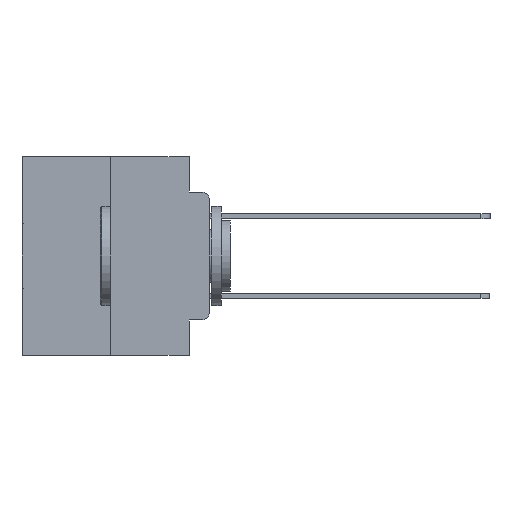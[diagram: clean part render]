
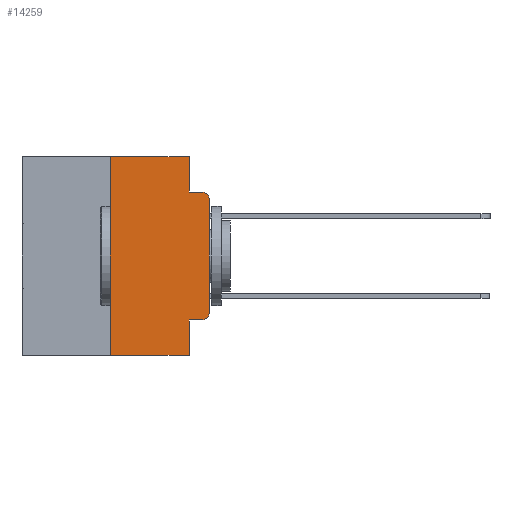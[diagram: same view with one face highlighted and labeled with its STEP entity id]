
A CAD part, left-side view. The second image highlights one B-rep face of the part: STEP entity #14259.
In plain terms, the highlighted planar face has unit normal (-1, 0, 0).
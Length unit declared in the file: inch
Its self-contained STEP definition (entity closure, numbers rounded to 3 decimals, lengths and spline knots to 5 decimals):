
#190 = LINE ( 'NONE', #10588, #1697 ) ;
#685 = CARTESIAN_POINT ( 'NONE',  ( 0., 0.051, -0.0885 ) ) ;
#853 = VERTEX_POINT ( 'NONE', #22486 ) ;
#1015 = EDGE_CURVE ( 'NONE', #21438, #19655, #23210, .T. ) ;
#1168 = VERTEX_POINT ( 'NONE', #1882 ) ;
#1697 = VECTOR ( 'NONE', #24722, 39.37008 ) ;
#1882 = CARTESIAN_POINT ( 'NONE',  ( 0., 0.25, 0. ) ) ;
#2859 = VECTOR ( 'NONE', #29440, 39.37008 ) ;
#3060 = LINE ( 'NONE', #21553, #28347 ) ;
#4230 = CARTESIAN_POINT ( 'NONE',  ( 0., 0.02, -0.3915 ) ) ;
#4765 = DIRECTION ( 'NONE',  ( 0., 0., -1. ) ) ;
#5165 = LINE ( 'NONE', #12017, #10908 ) ;
#5662 = EDGE_CURVE ( 'NONE', #25418, #853, #11537, .T. ) ;
#6187 = EDGE_CURVE ( 'NONE', #7221, #1168, #10761, .T. ) ;
#6679 = DIRECTION ( 'NONE',  ( 0., 0., -1. ) ) ;
#6810 = AXIS2_PLACEMENT_3D ( 'NONE', #12132, #28535, #14552 ) ;
#7221 = VERTEX_POINT ( 'NONE', #14687 ) ;
#7799 = CARTESIAN_POINT ( 'NONE',  ( 0., 0.473, -0.5 ) ) ;
#8168 = PLANE ( 'NONE',  #22833 ) ;
#8294 = CARTESIAN_POINT ( 'NONE',  ( 0., 0., -0.3915 ) ) ;
#9131 = CARTESIAN_POINT ( 'NONE',  ( 0., 0.02, -0.0885 ) ) ;
#9643 = ORIENTED_EDGE ( 'NONE', *, *, #25600, .T. ) ;
#9719 = DIRECTION ( 'NONE',  ( 0., -1., 0. ) ) ;
#9895 = VECTOR ( 'NONE', #11544, 39.37008 ) ;
#10014 = VECTOR ( 'NONE', #27582, 39.37008 ) ;
#10042 = ORIENTED_EDGE ( 'NONE', *, *, #19939, .F. ) ;
#10076 = ORIENTED_EDGE ( 'NONE', *, *, #5662, .T. ) ;
#10588 = CARTESIAN_POINT ( 'NONE',  ( 0., 0.051, 0. ) ) ;
#10681 = CARTESIAN_POINT ( 'NONE',  ( 0., 0.473, 0. ) ) ;
#10761 = LINE ( 'NONE', #13551, #10014 ) ;
#10908 = VECTOR ( 'NONE', #4765, 39.37008 ) ;
#11237 = ORIENTED_EDGE ( 'NONE', *, *, #11729, .T. ) ;
#11537 = LINE ( 'NONE', #25946, #29469 ) ;
#11544 = DIRECTION ( 'NONE',  ( 0., -1., 0. ) ) ;
#11729 = EDGE_CURVE ( 'NONE', #7221, #29117, #14611, .T. ) ;
#11973 = CARTESIAN_POINT ( 'NONE',  ( 0., 0.051, -0.4115 ) ) ;
#12017 = CARTESIAN_POINT ( 'NONE',  ( 0., 0.051, 0. ) ) ;
#12132 = CARTESIAN_POINT ( 'NONE',  ( 0., 0.02, -0.1085 ) ) ;
#12254 = EDGE_CURVE ( 'NONE', #853, #29142, #12320, .T. ) ;
#12320 = CIRCLE ( 'NONE', #6810, 0.02 ) ;
#13551 = CARTESIAN_POINT ( 'NONE',  ( 0., 0.25, 0. ) ) ;
#14259 = ADVANCED_FACE ( 'NONE', ( #22386 ), #8168, .F. ) ;
#14552 = DIRECTION ( 'NONE',  ( 0., 0., -1. ) ) ;
#14611 = LINE ( 'NONE', #7799, #20871 ) ;
#14687 = CARTESIAN_POINT ( 'NONE',  ( 0., 0.25, -0.5 ) ) ;
#14977 = EDGE_CURVE ( 'NONE', #1168, #20590, #22707, .T. ) ;
#15443 = DIRECTION ( 'NONE',  ( 0., 0., -1. ) ) ;
#17365 = CARTESIAN_POINT ( 'NONE',  ( 0., 0.051, -0.4115 ) ) ;
#18454 = EDGE_LOOP ( 'NONE', ( #10076, #27709, #10042, #28075, #29131, #24075, #11237, #23450, #20848, #9643 ) ) ;
#19655 = VERTEX_POINT ( 'NONE', #27514 ) ;
#19939 = EDGE_CURVE ( 'NONE', #24712, #29142, #3060, .T. ) ;
#20590 = VERTEX_POINT ( 'NONE', #28700 ) ;
#20848 = ORIENTED_EDGE ( 'NONE', *, *, #1015, .T. ) ;
#20871 = VECTOR ( 'NONE', #24416, 39.37008 ) ;
#21030 = DIRECTION ( 'NONE',  ( -1., 0., 0. ) ) ;
#21438 = VERTEX_POINT ( 'NONE', #11973 ) ;
#21553 = CARTESIAN_POINT ( 'NONE',  ( 0., 0.051, -0.0885 ) ) ;
#22385 = CIRCLE ( 'NONE', #24488, 0.02 ) ;
#22386 = FACE_OUTER_BOUND ( 'NONE', #18454, .T. ) ;
#22409 = CARTESIAN_POINT ( 'NONE',  ( 0., 0.473, 0. ) ) ;
#22486 = CARTESIAN_POINT ( 'NONE',  ( 0., 0., -0.1085 ) ) ;
#22707 = LINE ( 'NONE', #10681, #2859 ) ;
#22833 = AXIS2_PLACEMENT_3D ( 'NONE', #22409, #29383, #15443 ) ;
#23210 = LINE ( 'NONE', #17365, #9895 ) ;
#23450 = ORIENTED_EDGE ( 'NONE', *, *, #26580, .F. ) ;
#24075 = ORIENTED_EDGE ( 'NONE', *, *, #6187, .F. ) ;
#24416 = DIRECTION ( 'NONE',  ( 0., -1., 0. ) ) ;
#24488 = AXIS2_PLACEMENT_3D ( 'NONE', #4230, #21030, #6679 ) ;
#24712 = VERTEX_POINT ( 'NONE', #685 ) ;
#24722 = DIRECTION ( 'NONE',  ( 0., 0., -1. ) ) ;
#25418 = VERTEX_POINT ( 'NONE', #8294 ) ;
#25526 = CARTESIAN_POINT ( 'NONE',  ( 0., 0.051, -0.5 ) ) ;
#25600 = EDGE_CURVE ( 'NONE', #19655, #25418, #22385, .T. ) ;
#25753 = EDGE_CURVE ( 'NONE', #20590, #24712, #5165, .T. ) ;
#25946 = CARTESIAN_POINT ( 'NONE',  ( 0., 0., 0. ) ) ;
#26580 = EDGE_CURVE ( 'NONE', #21438, #29117, #190, .T. ) ;
#27514 = CARTESIAN_POINT ( 'NONE',  ( 0., 0.02, -0.4115 ) ) ;
#27582 = DIRECTION ( 'NONE',  ( 0., 0., 1. ) ) ;
#27709 = ORIENTED_EDGE ( 'NONE', *, *, #12254, .T. ) ;
#28075 = ORIENTED_EDGE ( 'NONE', *, *, #25753, .F. ) ;
#28347 = VECTOR ( 'NONE', #9719, 39.37008 ) ;
#28535 = DIRECTION ( 'NONE',  ( -1., 0., 0. ) ) ;
#28605 = DIRECTION ( 'NONE',  ( 0., 0., 1. ) ) ;
#28700 = CARTESIAN_POINT ( 'NONE',  ( 0., 0.051, 0. ) ) ;
#29117 = VERTEX_POINT ( 'NONE', #25526 ) ;
#29131 = ORIENTED_EDGE ( 'NONE', *, *, #14977, .F. ) ;
#29142 = VERTEX_POINT ( 'NONE', #9131 ) ;
#29383 = DIRECTION ( 'NONE',  ( 1., 0., 0. ) ) ;
#29440 = DIRECTION ( 'NONE',  ( 0., -1., 0. ) ) ;
#29469 = VECTOR ( 'NONE', #28605, 39.37008 ) ;
